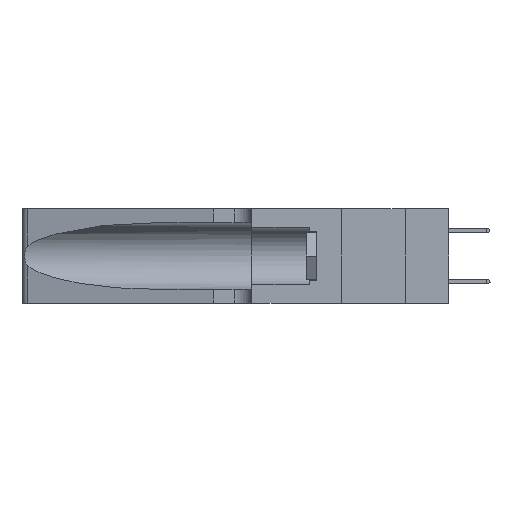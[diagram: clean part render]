
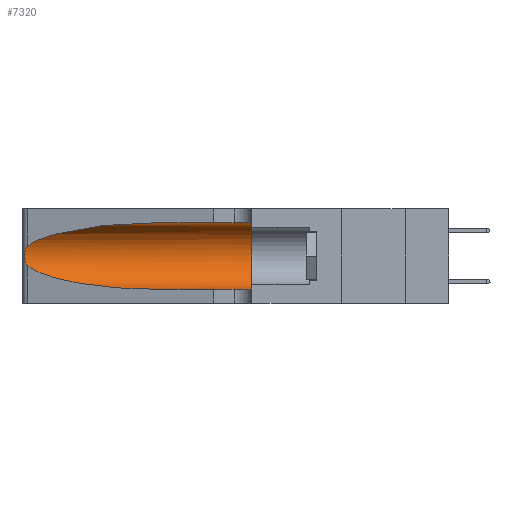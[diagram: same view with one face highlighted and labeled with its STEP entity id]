
A CAD part, left-side view. The second image highlights one B-rep face of the part: STEP entity #7320.
In plain terms, the highlighted cylindrical face has radius 3.308 mm (diameter 6.617 mm), a partial arc.
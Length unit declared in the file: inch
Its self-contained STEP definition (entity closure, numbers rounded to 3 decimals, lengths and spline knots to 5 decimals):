
#202 = CARTESIAN_POINT ( 'NONE',  ( 0.18966, 0.96281, 0.31525 ) ) ;
#416 = VERTEX_POINT ( 'NONE', #3197 ) ;
#480 = EDGE_CURVE ( 'NONE', #648, #7453, #12876, .T. ) ;
#499 = CARTESIAN_POINT ( 'NONE',  ( 0.25487, 1.22718, 0.22369 ) ) ;
#648 = VERTEX_POINT ( 'NONE', #4518 ) ;
#1089 = ORIENTED_EDGE ( 'NONE', *, *, #19859, .F. ) ;
#1448 = CARTESIAN_POINT ( 'NONE',  ( 0.1305, 1.61858, 0.05475 ) ) ;
#1561 = DIRECTION ( 'NONE',  ( 0., 0., -1. ) ) ;
#2205 = EDGE_CURVE ( 'NONE', #5695, #416, #9520, .T. ) ;
#2237 = CARTESIAN_POINT ( 'NONE',  ( 0.25487, 1.22718, 0.14631 ) ) ;
#2303 = CARTESIAN_POINT ( 'NONE',  ( 0.25555, 1.22994, 0.2215 ) ) ;
#2359 = EDGE_LOOP ( 'NONE', ( #16762, #5041, #11269, #18669, #3513, #1089 ) ) ;
#2376 = CARTESIAN_POINT ( 'NONE',  ( 0.26018, 1.23835, 0.19895 ) ) ;
#2456 = CARTESIAN_POINT ( 'NONE',  ( 0.25854, 1.2359, 0.20912 ) ) ;
#3077 = LINE ( 'NONE', #10321, #21368 ) ;
#3197 = CARTESIAN_POINT ( 'NONE',  ( 0.1305, 0.35, 0.05475 ) ) ;
#3345 = CARTESIAN_POINT ( 'NONE',  ( 0.1305, 1.61858, 0.185 ) ) ;
#3513 = ORIENTED_EDGE ( 'NONE', *, *, #14453, .F. ) ;
#3567 = DIRECTION ( 'NONE',  ( 0., -1., 0. ) ) ;
#3990 = CIRCLE ( 'NONE', #22438, 0.13025 ) ;
#4183 = CARTESIAN_POINT ( 'NONE',  ( 0.25856, 1.23593, 0.16098 ) ) ;
#4449 = AXIS2_PLACEMENT_3D ( 'NONE', #3345, #3567, #1561 ) ;
#4518 = CARTESIAN_POINT ( 'NONE',  ( 0.1305, 0.72297, 0.31525 ) ) ;
#5041 = ORIENTED_EDGE ( 'NONE', *, *, #20190, .T. ) ;
#5613 = CARTESIAN_POINT ( 'NONE',  ( 0.2373, 1.15595, 0.28018 ) ) ;
#5695 = VERTEX_POINT ( 'NONE', #7384 ) ;
#5908 = CARTESIAN_POINT ( 'NONE',  ( 0.26075, 1.23896, 0.19203 ) ) ;
#6544 = CARTESIAN_POINT ( 'NONE',  ( 0.1305, 0.35, 0.185 ) ) ;
#7320 = ADVANCED_FACE ( 'NONE', ( #20038 ), #7343, .F. ) ;
#7343 = CYLINDRICAL_SURFACE ( 'NONE', #4449, 0.13025 ) ;
#7384 = CARTESIAN_POINT ( 'NONE',  ( 0.1305, 0.72297, 0.05475 ) ) ;
#7453 = VERTEX_POINT ( 'NONE', #10833 ) ;
#7773 = CARTESIAN_POINT ( 'NONE',  ( 0.25789, 1.23486, 0.15765 ) ) ;
#8451 = VECTOR ( 'NONE', #8964, 39.37008 ) ;
#8964 = DIRECTION ( 'NONE',  ( 0., -1., 0. ) ) ;
#9172 = CARTESIAN_POINT ( 'NONE',  ( 0.1305, 0.35, 0.31525 ) ) ;
#9301 = CARTESIAN_POINT ( 'NONE',  ( 0.25787, 1.23484, 0.2124 ) ) ;
#9520 = LINE ( 'NONE', #1448, #8451 ) ;
#9534 = CARTESIAN_POINT ( 'NONE',  ( 0.25555, 1.22993, 0.14849 ) ) ;
#10321 = CARTESIAN_POINT ( 'NONE',  ( 0.1305, 1.61858, 0.31525 ) ) ;
#10693 = CARTESIAN_POINT ( 'NONE',  ( 0.18966, 0.96281, 0.05475 ) ) ;
#10833 = CARTESIAN_POINT ( 'NONE',  ( 0.25487, 1.22718, 0.22369 ) ) ;
#10839 = CARTESIAN_POINT ( 'NONE',  ( 0.1305, 0.72297, 0.05475 ) ) ;
#10909 = CARTESIAN_POINT ( 'NONE',  ( 0.25487, 1.22718, 0.22369 ) ) ;
#10911 = CARTESIAN_POINT ( 'NONE',  ( 0.25487, 1.22718, 0.14631 ) ) ;
#11027 = VERTEX_POINT ( 'NONE', #9172 ) ;
#11269 = ORIENTED_EDGE ( 'NONE', *, *, #19372, .T. ) ;
#11270 = CARTESIAN_POINT ( 'NONE',  ( 0.25487, 1.22718, 0.14631 ) ) ;
#12602 = CARTESIAN_POINT ( 'NONE',  ( 0.2373, 1.15595, 0.08982 ) ) ;
#12876 =( BOUNDED_CURVE ( )  B_SPLINE_CURVE ( 3, ( #16439, #202, #5613, #10909 ),
 .UNSPECIFIED., .F., .F. ) 
 B_SPLINE_CURVE_WITH_KNOTS ( ( 4, 4 ),
 ( 1.5708, 2.84003 ),
 .UNSPECIFIED. ) 
 CURVE ( )  GEOMETRIC_REPRESENTATION_ITEM ( )  RATIONAL_B_SPLINE_CURVE ( ( 1., 0.87, 0.87, 1. ) ) 
 REPRESENTATION_ITEM ( '' )  );
#13183 = DIRECTION ( 'NONE',  ( 0., 1., 0. ) ) ;
#13305 = VERTEX_POINT ( 'NONE', #2237 ) ;
#13915 =( BOUNDED_CURVE ( )  B_SPLINE_CURVE ( 3, ( #10911, #12602, #10693, #10839 ),
 .UNSPECIFIED., .F., .F. ) 
 B_SPLINE_CURVE_WITH_KNOTS ( ( 4, 4 ),
 ( 3.44316, 4.71239 ),
 .UNSPECIFIED. ) 
 CURVE ( )  GEOMETRIC_REPRESENTATION_ITEM ( )  RATIONAL_B_SPLINE_CURVE ( ( 1., 0.87, 0.87, 1. ) ) 
 REPRESENTATION_ITEM ( '' )  );
#14453 = EDGE_CURVE ( 'NONE', #11027, #416, #3990, .T. ) ;
#15666 = B_SPLINE_CURVE_WITH_KNOTS ( 'NONE', 3,
 ( #499, #2303, #18424, #9301, #2456, #2376, #5908, #18262, #20032, #4183, #7773, #20113, #9534, #11270 ),
 .UNSPECIFIED., .F., .F.,
 ( 4, 2, 2, 2, 2, 2, 4 ),
 ( 0., 0.00027, 0.00053, 0.00107, 0.0016, 0.00187, 0.00214 ),
 .UNSPECIFIED. ) ;
#15917 = DIRECTION ( 'NONE',  ( 0., -1., 0. ) ) ;
#16439 = CARTESIAN_POINT ( 'NONE',  ( 0.1305, 0.72297, 0.31525 ) ) ;
#16762 = ORIENTED_EDGE ( 'NONE', *, *, #480, .T. ) ;
#18262 = CARTESIAN_POINT ( 'NONE',  ( 0.26075, 1.23896, 0.178 ) ) ;
#18424 = CARTESIAN_POINT ( 'NONE',  ( 0.25639, 1.23184, 0.21858 ) ) ;
#18669 = ORIENTED_EDGE ( 'NONE', *, *, #2205, .T. ) ;
#19372 = EDGE_CURVE ( 'NONE', #13305, #5695, #13915, .T. ) ;
#19859 = EDGE_CURVE ( 'NONE', #648, #11027, #3077, .T. ) ;
#20032 = CARTESIAN_POINT ( 'NONE',  ( 0.26017, 1.23833, 0.17102 ) ) ;
#20038 = FACE_OUTER_BOUND ( 'NONE', #2359, .T. ) ;
#20113 = CARTESIAN_POINT ( 'NONE',  ( 0.25639, 1.23186, 0.15144 ) ) ;
#20190 = EDGE_CURVE ( 'NONE', #7453, #13305, #15666, .T. ) ;
#20586 = DIRECTION ( 'NONE',  ( 0., 0., 1. ) ) ;
#21368 = VECTOR ( 'NONE', #15917, 39.37008 ) ;
#22438 = AXIS2_PLACEMENT_3D ( 'NONE', #6544, #13183, #20586 ) ;
